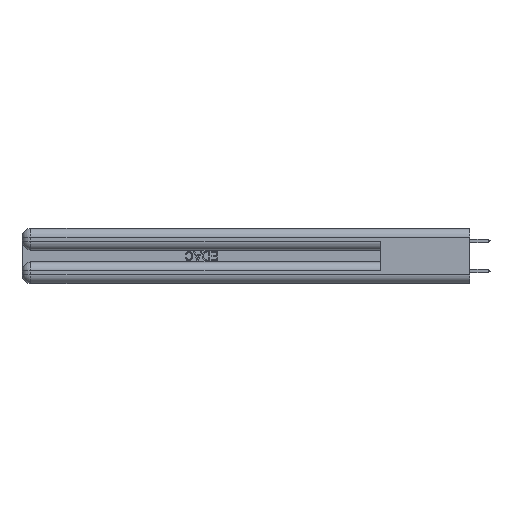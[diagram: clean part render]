
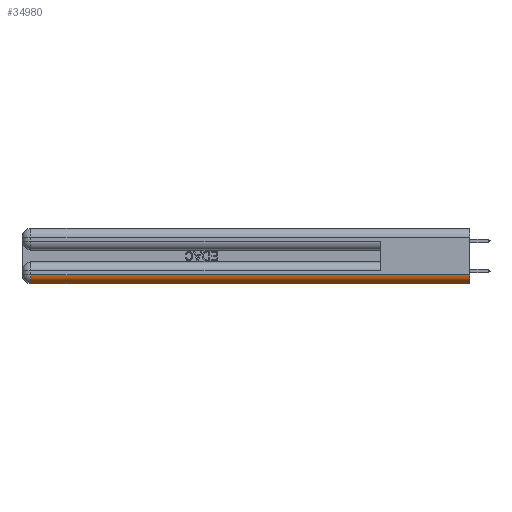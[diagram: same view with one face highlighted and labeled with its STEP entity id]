
A CAD part, left-side view. The second image highlights one B-rep face of the part: STEP entity #34980.
In plain terms, the highlighted cylindrical face has radius 1.524 mm (diameter 3.048 mm), a partial arc.
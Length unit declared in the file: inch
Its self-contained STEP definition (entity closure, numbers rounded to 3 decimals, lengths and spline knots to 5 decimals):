
#194 = CARTESIAN_POINT ( 'NONE',  ( 0.06, 0., 0. ) ) ;
#1210 = CARTESIAN_POINT ( 'NONE',  ( 0., 2.94, 0.06 ) ) ;
#2820 = VECTOR ( 'NONE', #15830, 39.37008 ) ;
#3655 = EDGE_CURVE ( 'NONE', #22343, #11020, #23776, .T. ) ;
#5124 = DIRECTION ( 'NONE',  ( 0., 0., 1. ) ) ;
#5533 = DIRECTION ( 'NONE',  ( 0., -1., 0. ) ) ;
#5951 = CARTESIAN_POINT ( 'NONE',  ( 0., 0., 0.06 ) ) ;
#6344 = DIRECTION ( 'NONE',  ( 0., 1., 0. ) ) ;
#7819 = AXIS2_PLACEMENT_3D ( 'NONE', #9856, #44122, #5124 ) ;
#9856 = CARTESIAN_POINT ( 'NONE',  ( 0.06, 0., 0.06 ) ) ;
#10061 = CARTESIAN_POINT ( 'NONE',  ( 0.06, 2.94, 0. ) ) ;
#11020 = VERTEX_POINT ( 'NONE', #1210 ) ;
#12740 = CIRCLE ( 'NONE', #7819, 0.06 ) ;
#15830 = DIRECTION ( 'NONE',  ( 0., 1., 0. ) ) ;
#19409 = DIRECTION ( 'NONE',  ( 0., 1., 0. ) ) ;
#19612 = VERTEX_POINT ( 'NONE', #5951 ) ;
#20040 = LINE ( 'NONE', #23098, #42255 ) ;
#20053 = CARTESIAN_POINT ( 'NONE',  ( 0.06, 2.94, 0.06 ) ) ;
#20108 = EDGE_CURVE ( 'NONE', #33931, #22343, #20619, .T. ) ;
#20602 = EDGE_CURVE ( 'NONE', #19612, #33931, #12740, .T. ) ;
#20619 = LINE ( 'NONE', #36277, #2820 ) ;
#22343 = VERTEX_POINT ( 'NONE', #10061 ) ;
#23098 = CARTESIAN_POINT ( 'NONE',  ( 0., 0., 0.06 ) ) ;
#23464 = AXIS2_PLACEMENT_3D ( 'NONE', #31218, #6344, #42064 ) ;
#23776 = CIRCLE ( 'NONE', #29813, 0.06 ) ;
#27754 = CYLINDRICAL_SURFACE ( 'NONE', #23464, 0.06 ) ;
#29813 = AXIS2_PLACEMENT_3D ( 'NONE', #20053, #19409, #44581 ) ;
#31218 = CARTESIAN_POINT ( 'NONE',  ( 0.06, 0., 0.06 ) ) ;
#31628 = FACE_OUTER_BOUND ( 'NONE', #45047, .T. ) ;
#33464 = ORIENTED_EDGE ( 'NONE', *, *, #33611, .F. ) ;
#33611 = EDGE_CURVE ( 'NONE', #11020, #19612, #20040, .T. ) ;
#33931 = VERTEX_POINT ( 'NONE', #194 ) ;
#34980 = ADVANCED_FACE ( 'NONE', ( #31628 ), #27754, .T. ) ;
#35025 = ORIENTED_EDGE ( 'NONE', *, *, #20602, .F. ) ;
#36277 = CARTESIAN_POINT ( 'NONE',  ( 0.06, 3., 0. ) ) ;
#38656 = ORIENTED_EDGE ( 'NONE', *, *, #3655, .F. ) ;
#42064 = DIRECTION ( 'NONE',  ( 0., 0., 1. ) ) ;
#42255 = VECTOR ( 'NONE', #5533, 39.37008 ) ;
#44122 = DIRECTION ( 'NONE',  ( 0., -1., 0. ) ) ;
#44346 = ORIENTED_EDGE ( 'NONE', *, *, #20108, .F. ) ;
#44581 = DIRECTION ( 'NONE',  ( 0., 0., 1. ) ) ;
#45047 = EDGE_LOOP ( 'NONE', ( #35025, #33464, #38656, #44346 ) ) ;
